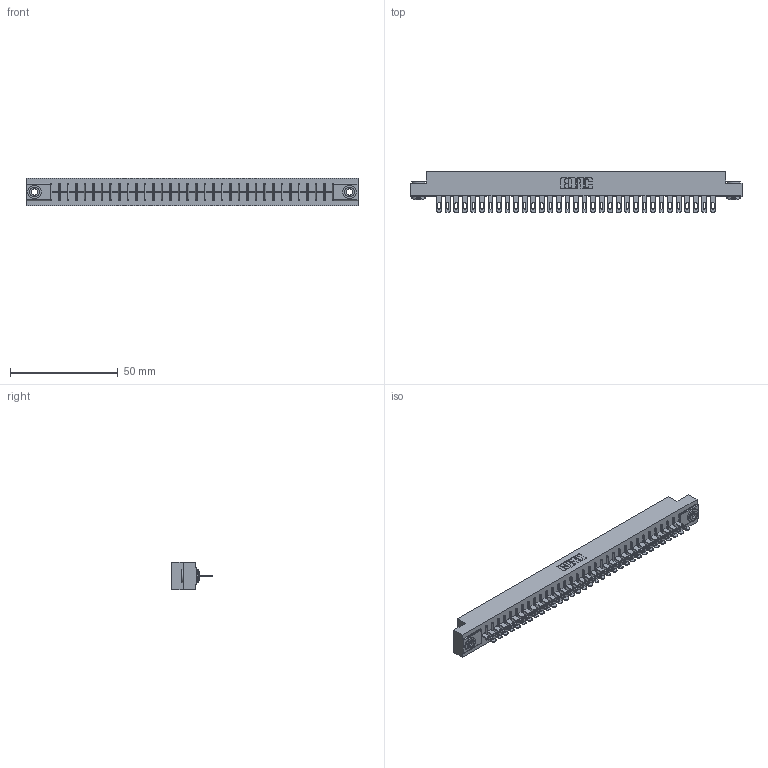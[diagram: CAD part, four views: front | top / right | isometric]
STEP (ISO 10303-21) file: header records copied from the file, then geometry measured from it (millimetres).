
FILE_DESCRIPTION (( 'STEP AP203' ), '1' );
FILE_NAME ('306-033-500-103.STEP', '2019-09-11T22:51:50', ( '' ), ( '' ), 'SwSTEP 2.0', 'SolidWorks 2016', '' );
FILE_SCHEMA (( 'CONFIG_CONTROL_DESIGN' ));
Length unit declared in the file: inch
Products named in the file (4): 306-033-500-103; 345-250-002_345-250-002-102; 306 Part_.156 Dia; 306-290-001_100
Assembly tree (36 placements, depth 2):
  306-033-500-103
    306 Part_.156 Dia
    306-290-001_100  x33
    345-250-002_345-250-002-102  x2
Bounding box: 153.77 x 18.87 x 12.7 mm (x, y, z)
Volume: 17028.6 mm3; surface area: 18220.8 mm2
Topology: 36 solids, 36 shells, 2676 faces, 7523 edges, 4834 vertices
Faces by surface type: plane 1742, cylinder 794, sphere 132, cone 8
Entity records: 33169 total; most frequent: CARTESIAN_POINT 5547, ORIENTED_EDGE 5490, DIRECTION 5485, EDGE_CURVE 2745, VECTOR 2133, LINE 2133, VERTEX_POINT 1738, AXIS2_PLACEMENT_3D 1676
